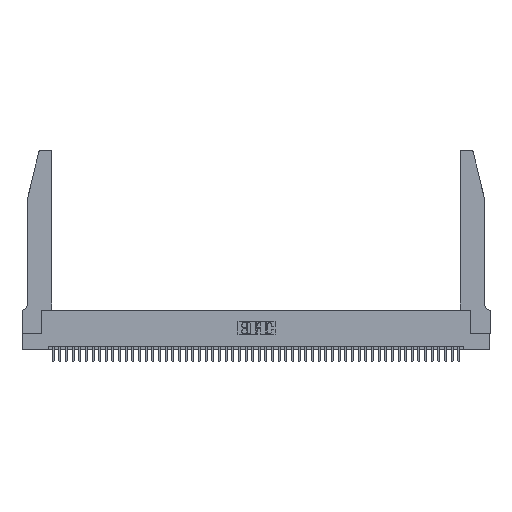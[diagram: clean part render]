
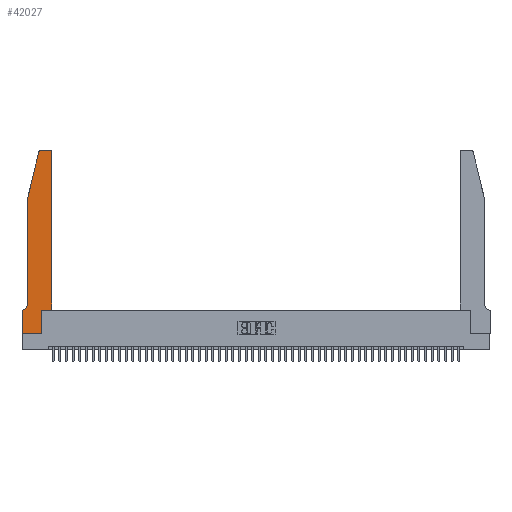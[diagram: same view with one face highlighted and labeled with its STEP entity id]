
A CAD part, top view. The second image highlights one B-rep face of the part: STEP entity #42027.
In plain terms, the highlighted planar face has unit normal (0, 0, 1).
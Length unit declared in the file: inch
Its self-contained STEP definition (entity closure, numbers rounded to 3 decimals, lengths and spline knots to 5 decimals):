
#1310 = ORIENTED_EDGE ( 'NONE', *, *, #10210, .T. ) ;
#1450 = EDGE_CURVE ( 'NONE', #43237, #12546, #4770, .T. ) ;
#2244 = VERTEX_POINT ( 'NONE', #13887 ) ;
#2437 = DIRECTION ( 'NONE',  ( 1., 0., 0. ) ) ;
#2817 = EDGE_CURVE ( 'NONE', #23635, #50776, #33174, .T. ) ;
#3127 = CARTESIAN_POINT ( 'NONE',  ( 0.4505, 0.35, 0.37 ) ) ;
#3193 = CARTESIAN_POINT ( 'NONE',  ( 0.284, 2.75, 0.37 ) ) ;
#3396 = CARTESIAN_POINT ( 'NONE',  ( 0., 0.35, 0.37 ) ) ;
#4770 = CIRCLE ( 'NONE', #44121, 0.03 ) ;
#5379 = DIRECTION ( 'NONE',  ( -1., 0., 0. ) ) ;
#5806 = VECTOR ( 'NONE', #36749, 39.37008 ) ;
#8637 = VERTEX_POINT ( 'NONE', #28885 ) ;
#8877 = CARTESIAN_POINT ( 'NONE',  ( 0.25487, 2.72718, 0.37 ) ) ;
#9181 = CARTESIAN_POINT ( 'NONE',  ( 0., 0., 0.37 ) ) ;
#9818 = DIRECTION ( 'NONE',  ( 0., 0., 1. ) ) ;
#9829 = ORIENTED_EDGE ( 'NONE', *, *, #37308, .T. ) ;
#10084 = CARTESIAN_POINT ( 'NONE',  ( 0.2865, 0.35, 0.37 ) ) ;
#10210 = EDGE_CURVE ( 'NONE', #50776, #43237, #14322, .T. ) ;
#10256 = PLANE ( 'NONE',  #38664 ) ;
#11211 = EDGE_CURVE ( 'NONE', #28242, #8637, #45517, .T. ) ;
#11689 = ORIENTED_EDGE ( 'NONE', *, *, #24084, .T. ) ;
#12088 = CARTESIAN_POINT ( 'NONE',  ( 0.2605, 2.75, 0.37 ) ) ;
#12546 = VERTEX_POINT ( 'NONE', #8877 ) ;
#12606 = VERTEX_POINT ( 'NONE', #24783 ) ;
#13113 = EDGE_CURVE ( 'NONE', #40712, #2244, #32560, .T. ) ;
#13401 = CARTESIAN_POINT ( 'NONE',  ( 0.0755, 0.35, 0.37 ) ) ;
#13478 = ORIENTED_EDGE ( 'NONE', *, *, #11211, .T. ) ;
#13601 = DIRECTION ( 'NONE',  ( 0., 0., 1. ) ) ;
#13750 = AXIS2_PLACEMENT_3D ( 'NONE', #16900, #44369, #20862 ) ;
#13887 = CARTESIAN_POINT ( 'NONE',  ( 0.2865, 0., 0.37 ) ) ;
#14322 = LINE ( 'NONE', #12088, #34058 ) ;
#14606 = EDGE_LOOP ( 'NONE', ( #1310, #27780, #9829, #25919, #11689, #44868, #20306, #15345, #18414, #13478, #50150, #22100 ) ) ;
#15345 = ORIENTED_EDGE ( 'NONE', *, *, #13113, .T. ) ;
#16900 = CARTESIAN_POINT ( 'NONE',  ( 0.0055, 0.42, 0.37 ) ) ;
#16951 = VERTEX_POINT ( 'NONE', #19402 ) ;
#18142 = CARTESIAN_POINT ( 'NONE',  ( 0.4505, 2.72, 0.37 ) ) ;
#18414 = ORIENTED_EDGE ( 'NONE', *, *, #38876, .T. ) ;
#18940 = CARTESIAN_POINT ( 'NONE',  ( 0.4505, 0.35, 0.37 ) ) ;
#19402 = CARTESIAN_POINT ( 'NONE',  ( 0.0755, 0.42, 0.37 ) ) ;
#19885 = DIRECTION ( 'NONE',  ( 1., 0., 0. ) ) ;
#20191 = CARTESIAN_POINT ( 'NONE',  ( 0.4205, 2.75, 0.37 ) ) ;
#20306 = ORIENTED_EDGE ( 'NONE', *, *, #24661, .T. ) ;
#20716 = VECTOR ( 'NONE', #5379, 39.37008 ) ;
#20862 = DIRECTION ( 'NONE',  ( -1., 0., 0. ) ) ;
#22100 = ORIENTED_EDGE ( 'NONE', *, *, #2817, .T. ) ;
#23150 = VECTOR ( 'NONE', #26879, 39.37008 ) ;
#23635 = VERTEX_POINT ( 'NONE', #18142 ) ;
#24084 = EDGE_CURVE ( 'NONE', #16951, #12606, #39801, .T. ) ;
#24661 = EDGE_CURVE ( 'NONE', #29880, #40712, #36076, .T. ) ;
#24783 = CARTESIAN_POINT ( 'NONE',  ( 0.0055, 0.35, 0.37 ) ) ;
#24938 = VERTEX_POINT ( 'NONE', #26623 ) ;
#25919 = ORIENTED_EDGE ( 'NONE', *, *, #36421, .T. ) ;
#26132 = CARTESIAN_POINT ( 'NONE',  ( 0., 0., 0.37 ) ) ;
#26184 = DIRECTION ( 'NONE',  ( 0., 0., 1. ) ) ;
#26623 = CARTESIAN_POINT ( 'NONE',  ( 0.0755, 2., 0.37 ) ) ;
#26879 = DIRECTION ( 'NONE',  ( 0., 1., 0. ) ) ;
#27331 = VECTOR ( 'NONE', #28204, 39.37008 ) ;
#27780 = ORIENTED_EDGE ( 'NONE', *, *, #1450, .T. ) ;
#27825 = CARTESIAN_POINT ( 'NONE',  ( 0., 0., 0.37 ) ) ;
#28204 = DIRECTION ( 'NONE',  ( -0.239, -0.971, 0. ) ) ;
#28242 = VERTEX_POINT ( 'NONE', #44716 ) ;
#28885 = CARTESIAN_POINT ( 'NONE',  ( 0.4505, 0.35, 0.37 ) ) ;
#29880 = VERTEX_POINT ( 'NONE', #3396 ) ;
#29899 = LINE ( 'NONE', #42443, #39062 ) ;
#30685 = DIRECTION ( 'NONE',  ( 0., -1., 0. ) ) ;
#32560 = LINE ( 'NONE', #27825, #41681 ) ;
#33174 = CIRCLE ( 'NONE', #40229, 0.03 ) ;
#33491 = CARTESIAN_POINT ( 'NONE',  ( 0.4205, 2.72, 0.37 ) ) ;
#34058 = VECTOR ( 'NONE', #39623, 39.37008 ) ;
#34338 = FACE_OUTER_BOUND ( 'NONE', #14606, .T. ) ;
#34612 = DIRECTION ( 'NONE',  ( 1., 0., 0. ) ) ;
#34760 = EDGE_CURVE ( 'NONE', #12606, #29880, #41594, .T. ) ;
#35910 = CARTESIAN_POINT ( 'NONE',  ( 0.0755, 2., 0.37 ) ) ;
#36076 = LINE ( 'NONE', #9181, #5806 ) ;
#36421 = EDGE_CURVE ( 'NONE', #24938, #16951, #29899, .T. ) ;
#36749 = DIRECTION ( 'NONE',  ( 0., -1., 0. ) ) ;
#37167 = CARTESIAN_POINT ( 'NONE',  ( 0.284, 2.72, 0.37 ) ) ;
#37308 = EDGE_CURVE ( 'NONE', #12546, #24938, #48032, .T. ) ;
#37385 = DIRECTION ( 'NONE',  ( 1., 0., 0. ) ) ;
#38177 = LINE ( 'NONE', #10084, #39410 ) ;
#38664 = AXIS2_PLACEMENT_3D ( 'NONE', #49452, #26184, #2437 ) ;
#38876 = EDGE_CURVE ( 'NONE', #2244, #28242, #38177, .T. ) ;
#39062 = VECTOR ( 'NONE', #30685, 39.37008 ) ;
#39410 = VECTOR ( 'NONE', #41559, 39.37008 ) ;
#39623 = DIRECTION ( 'NONE',  ( -1., 0., 0. ) ) ;
#39801 = CIRCLE ( 'NONE', #13750, 0.07 ) ;
#40229 = AXIS2_PLACEMENT_3D ( 'NONE', #33491, #9818, #37385 ) ;
#40712 = VERTEX_POINT ( 'NONE', #26132 ) ;
#41096 = DIRECTION ( 'NONE',  ( 1., 0., 0. ) ) ;
#41559 = DIRECTION ( 'NONE',  ( 0., 1., 0. ) ) ;
#41594 = LINE ( 'NONE', #13401, #20716 ) ;
#41681 = VECTOR ( 'NONE', #19885, 39.37008 ) ;
#42027 = ADVANCED_FACE ( 'NONE', ( #34338 ), #10256, .T. ) ;
#42443 = CARTESIAN_POINT ( 'NONE',  ( 0.0755, 2., 0.37 ) ) ;
#42756 = LINE ( 'NONE', #3127, #23150 ) ;
#43099 = VECTOR ( 'NONE', #34612, 39.37008 ) ;
#43237 = VERTEX_POINT ( 'NONE', #3193 ) ;
#43870 = EDGE_CURVE ( 'NONE', #8637, #23635, #42756, .T. ) ;
#44121 = AXIS2_PLACEMENT_3D ( 'NONE', #37167, #13601, #41096 ) ;
#44369 = DIRECTION ( 'NONE',  ( 0., 0., -1. ) ) ;
#44716 = CARTESIAN_POINT ( 'NONE',  ( 0.2865, 0.35, 0.37 ) ) ;
#44868 = ORIENTED_EDGE ( 'NONE', *, *, #34760, .T. ) ;
#45517 = LINE ( 'NONE', #18940, #43099 ) ;
#48032 = LINE ( 'NONE', #35910, #27331 ) ;
#49452 = CARTESIAN_POINT ( 'NONE',  ( 0., 0.35, 0.37 ) ) ;
#50150 = ORIENTED_EDGE ( 'NONE', *, *, #43870, .T. ) ;
#50776 = VERTEX_POINT ( 'NONE', #20191 ) ;
